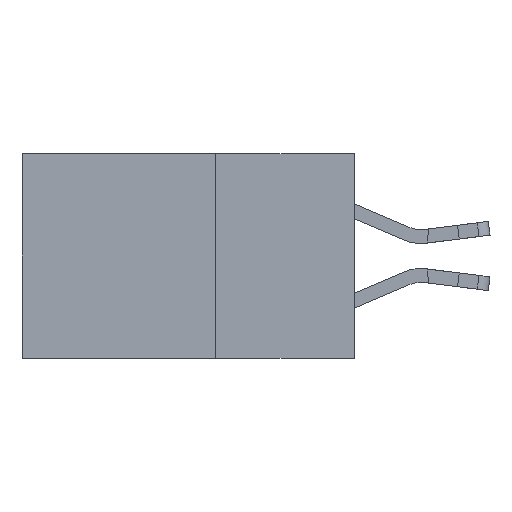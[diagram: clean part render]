
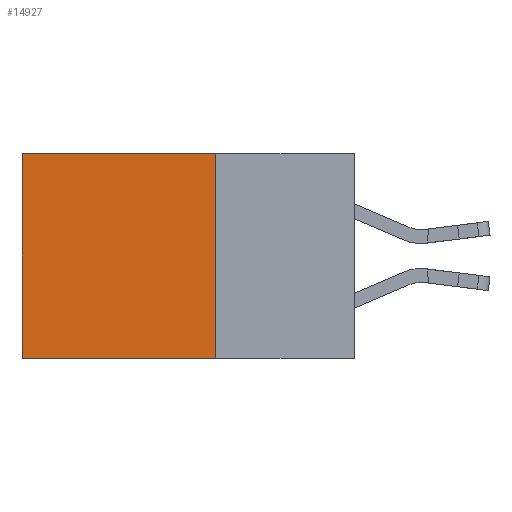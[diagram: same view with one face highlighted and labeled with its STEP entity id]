
A CAD part, left-side view. The second image highlights one B-rep face of the part: STEP entity #14927.
In plain terms, the highlighted planar face has unit normal (-1, 0, 0).
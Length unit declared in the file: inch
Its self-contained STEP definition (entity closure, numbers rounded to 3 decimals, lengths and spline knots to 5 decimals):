
#857 = CARTESIAN_POINT ( 'NONE',  ( 0.298, 0.25, 0. ) ) ;
#1303 = FACE_OUTER_BOUND ( 'NONE', #4352, .T. ) ;
#1615 = CARTESIAN_POINT ( 'NONE',  ( 0.298, 0.25, -0.37 ) ) ;
#2507 = LINE ( 'NONE', #10060, #10159 ) ;
#2603 = DIRECTION ( 'NONE',  ( 0., 0., -1. ) ) ;
#2757 = VERTEX_POINT ( 'NONE', #15921 ) ;
#3491 = VERTEX_POINT ( 'NONE', #11883 ) ;
#3706 = ORIENTED_EDGE ( 'NONE', *, *, #17571, .T. ) ;
#4352 = EDGE_LOOP ( 'NONE', ( #3706, #4707, #13085, #5935 ) ) ;
#4707 = ORIENTED_EDGE ( 'NONE', *, *, #15075, .F. ) ;
#4978 = LINE ( 'NONE', #17516, #8539 ) ;
#5170 = DIRECTION ( 'NONE',  ( 0., 0., -1. ) ) ;
#5532 = DIRECTION ( 'NONE',  ( 0., 1., 0. ) ) ;
#5935 = ORIENTED_EDGE ( 'NONE', *, *, #13804, .T. ) ;
#6645 = LINE ( 'NONE', #857, #18443 ) ;
#8539 = VECTOR ( 'NONE', #2603, 39.37008 ) ;
#9038 = VERTEX_POINT ( 'NONE', #1615 ) ;
#9678 = CARTESIAN_POINT ( 'NONE',  ( 0.298, 0.25, 0. ) ) ;
#10060 = CARTESIAN_POINT ( 'NONE',  ( 0.298, 0.25, -0.37 ) ) ;
#10159 = VECTOR ( 'NONE', #11614, 39.37008 ) ;
#10675 = CARTESIAN_POINT ( 'NONE',  ( 0.298, 0.6, 0. ) ) ;
#11614 = DIRECTION ( 'NONE',  ( 0., 1., 0. ) ) ;
#11883 = CARTESIAN_POINT ( 'NONE',  ( 0.298, 0.25, 0. ) ) ;
#12699 = PLANE ( 'NONE',  #17407 ) ;
#13085 = ORIENTED_EDGE ( 'NONE', *, *, #14522, .F. ) ;
#13801 = VECTOR ( 'NONE', #17529, 39.37008 ) ;
#13804 = EDGE_CURVE ( 'NONE', #3491, #15340, #6645, .T. ) ;
#14149 = DIRECTION ( 'NONE',  ( 1., 0., 0. ) ) ;
#14427 = CARTESIAN_POINT ( 'NONE',  ( 0.298, 0.6, 0. ) ) ;
#14522 = EDGE_CURVE ( 'NONE', #3491, #9038, #4978, .T. ) ;
#14927 = ADVANCED_FACE ( 'NONE', ( #1303 ), #12699, .F. ) ;
#15075 = EDGE_CURVE ( 'NONE', #9038, #2757, #2507, .T. ) ;
#15340 = VERTEX_POINT ( 'NONE', #10675 ) ;
#15921 = CARTESIAN_POINT ( 'NONE',  ( 0.298, 0.6, -0.37 ) ) ;
#17407 = AXIS2_PLACEMENT_3D ( 'NONE', #9678, #14149, #5170 ) ;
#17516 = CARTESIAN_POINT ( 'NONE',  ( 0.298, 0.25, 0. ) ) ;
#17529 = DIRECTION ( 'NONE',  ( 0., 0., -1. ) ) ;
#17571 = EDGE_CURVE ( 'NONE', #15340, #2757, #17637, .T. ) ;
#17637 = LINE ( 'NONE', #14427, #13801 ) ;
#18443 = VECTOR ( 'NONE', #5532, 39.37008 ) ;
